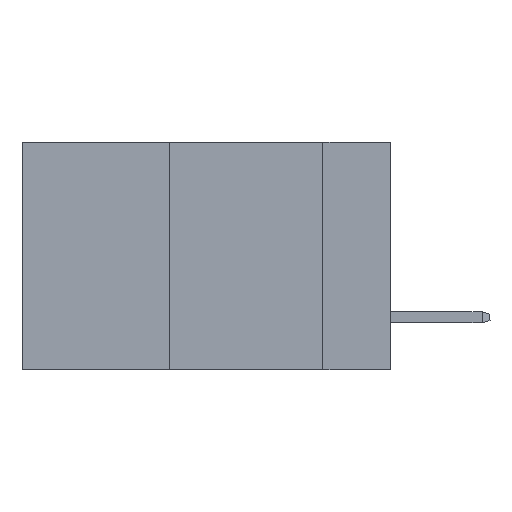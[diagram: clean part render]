
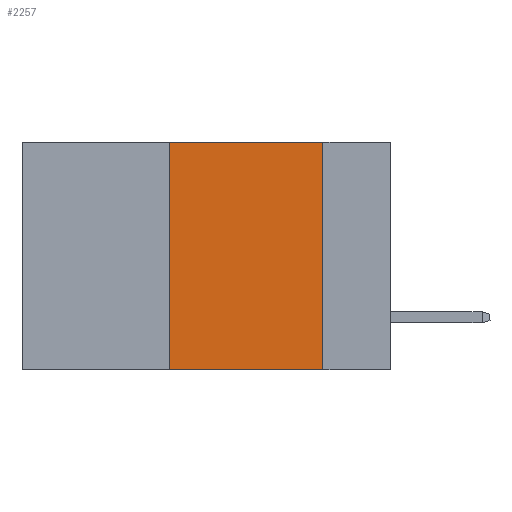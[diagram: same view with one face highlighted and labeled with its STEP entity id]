
A CAD part, left-side view. The second image highlights one B-rep face of the part: STEP entity #2257.
In plain terms, the highlighted planar face has unit normal (-1, 0, 0).
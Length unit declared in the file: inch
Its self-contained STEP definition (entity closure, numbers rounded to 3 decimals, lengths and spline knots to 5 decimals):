
#1329 = VERTEX_POINT ( 'NONE', #5467 ) ;
#1420 = CARTESIAN_POINT ( 'NONE',  ( 0., 0.6, 0. ) ) ;
#1578 = LINE ( 'NONE', #8359, #10914 ) ;
#1803 = DIRECTION ( 'NONE',  ( 0., 0., -1. ) ) ;
#1824 = EDGE_CURVE ( 'NONE', #1870, #3944, #2805, .T. ) ;
#1870 = VERTEX_POINT ( 'NONE', #11070 ) ;
#2037 = VECTOR ( 'NONE', #10446, 39.37008 ) ;
#2257 = ADVANCED_FACE ( 'NONE', ( #3380 ), #11137, .F. ) ;
#2805 = LINE ( 'NONE', #1420, #7292 ) ;
#3380 = FACE_OUTER_BOUND ( 'NONE', #6406, .T. ) ;
#3594 = EDGE_CURVE ( 'NONE', #10915, #1870, #1578, .T. ) ;
#3800 = CARTESIAN_POINT ( 'NONE',  ( 0., 0.6, 0. ) ) ;
#3843 = DIRECTION ( 'NONE',  ( 1., 0., 0. ) ) ;
#3944 = VERTEX_POINT ( 'NONE', #11079 ) ;
#3948 = DIRECTION ( 'NONE',  ( 0., -1., 0. ) ) ;
#4377 = AXIS2_PLACEMENT_3D ( 'NONE', #3800, #3843, #1803 ) ;
#4450 = CARTESIAN_POINT ( 'NONE',  ( 0., 0.6, -0.37 ) ) ;
#5324 = DIRECTION ( 'NONE',  ( 0., 0., -1. ) ) ;
#5467 = CARTESIAN_POINT ( 'NONE',  ( 0., 0.11, -0.37 ) ) ;
#5498 = LINE ( 'NONE', #9620, #9794 ) ;
#5827 = DIRECTION ( 'NONE',  ( 0., 0., 1. ) ) ;
#6406 = EDGE_LOOP ( 'NONE', ( #9113, #11395, #7601, #10214 ) ) ;
#7292 = VECTOR ( 'NONE', #3948, 39.37008 ) ;
#7534 = EDGE_CURVE ( 'NONE', #3944, #1329, #5498, .T. ) ;
#7601 = ORIENTED_EDGE ( 'NONE', *, *, #3594, .F. ) ;
#8359 = CARTESIAN_POINT ( 'NONE',  ( 0., 0.36, 0. ) ) ;
#8865 = LINE ( 'NONE', #4450, #2037 ) ;
#9113 = ORIENTED_EDGE ( 'NONE', *, *, #7534, .F. ) ;
#9564 = CARTESIAN_POINT ( 'NONE',  ( 0., 0.36, -0.37 ) ) ;
#9620 = CARTESIAN_POINT ( 'NONE',  ( 0., 0.11, 0. ) ) ;
#9794 = VECTOR ( 'NONE', #5324, 39.37008 ) ;
#10214 = ORIENTED_EDGE ( 'NONE', *, *, #10392, .T. ) ;
#10392 = EDGE_CURVE ( 'NONE', #10915, #1329, #8865, .T. ) ;
#10446 = DIRECTION ( 'NONE',  ( 0., -1., 0. ) ) ;
#10914 = VECTOR ( 'NONE', #5827, 39.37008 ) ;
#10915 = VERTEX_POINT ( 'NONE', #9564 ) ;
#11070 = CARTESIAN_POINT ( 'NONE',  ( 0., 0.36, 0. ) ) ;
#11079 = CARTESIAN_POINT ( 'NONE',  ( 0., 0.11, 0. ) ) ;
#11137 = PLANE ( 'NONE',  #4377 ) ;
#11395 = ORIENTED_EDGE ( 'NONE', *, *, #1824, .F. ) ;
